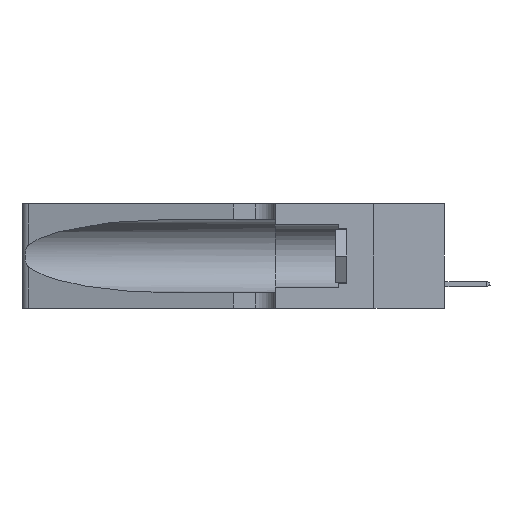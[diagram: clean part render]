
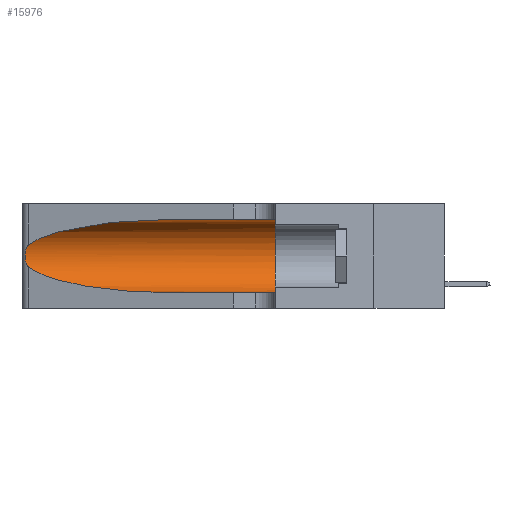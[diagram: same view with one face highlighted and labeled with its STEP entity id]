
A CAD part, left-side view. The second image highlights one B-rep face of the part: STEP entity #15976.
In plain terms, the highlighted cylindrical face has radius 3.308 mm (diameter 6.617 mm), a partial arc.
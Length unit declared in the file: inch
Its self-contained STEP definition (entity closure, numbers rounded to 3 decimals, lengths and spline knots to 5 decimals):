
#788 = CARTESIAN_POINT ( 'NONE',  ( 0.25487, 1.22718, 0.22369 ) ) ;
#1173 = CARTESIAN_POINT ( 'NONE',  ( 0.1305, 0.72297, 0.05475 ) ) ;
#1463 = DIRECTION ( 'NONE',  ( 0., -1., 0. ) ) ;
#1502 = CARTESIAN_POINT ( 'NONE',  ( 0.26018, 1.23835, 0.19895 ) ) ;
#1537 = ORIENTED_EDGE ( 'NONE', *, *, #6121, .T. ) ;
#1835 = VERTEX_POINT ( 'NONE', #3418 ) ;
#2239 = B_SPLINE_CURVE_WITH_KNOTS ( 'NONE', 3,
 ( #13172, #17403, #13436, #3181, #11538, #1502, #15188, #3264, #3517, #17482, #17229, #19241, #7269, #13515 ),
 .UNSPECIFIED., .F., .F.,
 ( 4, 2, 2, 2, 2, 2, 4 ),
 ( 0., 0.00027, 0.00053, 0.00107, 0.0016, 0.00187, 0.00214 ),
 .UNSPECIFIED. ) ;
#2704 = CARTESIAN_POINT ( 'NONE',  ( 0.2373, 1.15595, 0.08982 ) ) ;
#2873 = CARTESIAN_POINT ( 'NONE',  ( 0.25487, 1.22718, 0.14631 ) ) ;
#3123 = VERTEX_POINT ( 'NONE', #2873 ) ;
#3129 = VECTOR ( 'NONE', #4085, 39.37008 ) ;
#3181 = CARTESIAN_POINT ( 'NONE',  ( 0.25787, 1.23484, 0.2124 ) ) ;
#3264 = CARTESIAN_POINT ( 'NONE',  ( 0.26075, 1.23896, 0.178 ) ) ;
#3418 = CARTESIAN_POINT ( 'NONE',  ( 0.1305, 0.35, 0.05475 ) ) ;
#3517 = CARTESIAN_POINT ( 'NONE',  ( 0.26017, 1.23833, 0.17102 ) ) ;
#3657 = CARTESIAN_POINT ( 'NONE',  ( 0.1305, 0.35, 0.185 ) ) ;
#4085 = DIRECTION ( 'NONE',  ( 0., -1., 0. ) ) ;
#4958 = CARTESIAN_POINT ( 'NONE',  ( 0.18966, 0.96281, 0.31525 ) ) ;
#5307 = EDGE_CURVE ( 'NONE', #25484, #12377, #20022, .T. ) ;
#5622 = DIRECTION ( 'NONE',  ( 0., 1., 0. ) ) ;
#6121 = EDGE_CURVE ( 'NONE', #3123, #25502, #10737, .T. ) ;
#6698 = CARTESIAN_POINT ( 'NONE',  ( 0.18966, 0.96281, 0.05475 ) ) ;
#6834 = EDGE_CURVE ( 'NONE', #12377, #3123, #2239, .T. ) ;
#6978 = CARTESIAN_POINT ( 'NONE',  ( 0.2373, 1.15595, 0.28018 ) ) ;
#7135 = VECTOR ( 'NONE', #20220, 39.37008 ) ;
#7269 = CARTESIAN_POINT ( 'NONE',  ( 0.25555, 1.22993, 0.14849 ) ) ;
#7439 = LINE ( 'NONE', #25534, #7135 ) ;
#7719 = DIRECTION ( 'NONE',  ( 0., 0., 1. ) ) ;
#7874 = ORIENTED_EDGE ( 'NONE', *, *, #12235, .F. ) ;
#8394 = LINE ( 'NONE', #21883, #3129 ) ;
#8691 = CARTESIAN_POINT ( 'NONE',  ( 0.1305, 0.72297, 0.05475 ) ) ;
#10331 = EDGE_CURVE ( 'NONE', #25484, #12936, #8394, .T. ) ;
#10737 =( BOUNDED_CURVE ( )  B_SPLINE_CURVE ( 3, ( #25036, #2704, #6698, #8691 ),
 .UNSPECIFIED., .F., .T. ) 
 B_SPLINE_CURVE_WITH_KNOTS ( ( 4, 4 ),
 ( 3.44316, 4.71239 ),
 .UNSPECIFIED. ) 
 CURVE ( )  GEOMETRIC_REPRESENTATION_ITEM ( )  RATIONAL_B_SPLINE_CURVE ( ( 1., 0.87, 0.87, 1. ) ) 
 REPRESENTATION_ITEM ( '' )  );
#11096 = CARTESIAN_POINT ( 'NONE',  ( 0.1305, 0.72297, 0.31525 ) ) ;
#11343 = CARTESIAN_POINT ( 'NONE',  ( 0.25487, 1.22718, 0.22369 ) ) ;
#11538 = CARTESIAN_POINT ( 'NONE',  ( 0.25854, 1.2359, 0.20912 ) ) ;
#11577 = CARTESIAN_POINT ( 'NONE',  ( 0.1305, 1.61858, 0.185 ) ) ;
#11634 = CYLINDRICAL_SURFACE ( 'NONE', #13107, 0.13025 ) ;
#12021 = EDGE_CURVE ( 'NONE', #25502, #1835, #7439, .T. ) ;
#12235 = EDGE_CURVE ( 'NONE', #12936, #1835, #13033, .T. ) ;
#12252 = FACE_OUTER_BOUND ( 'NONE', #20084, .T. ) ;
#12377 = VERTEX_POINT ( 'NONE', #788 ) ;
#12936 = VERTEX_POINT ( 'NONE', #19093 ) ;
#13033 = CIRCLE ( 'NONE', #22105, 0.13025 ) ;
#13107 = AXIS2_PLACEMENT_3D ( 'NONE', #11577, #1463, #23694 ) ;
#13172 = CARTESIAN_POINT ( 'NONE',  ( 0.25487, 1.22718, 0.22369 ) ) ;
#13436 = CARTESIAN_POINT ( 'NONE',  ( 0.25639, 1.23184, 0.21858 ) ) ;
#13515 = CARTESIAN_POINT ( 'NONE',  ( 0.25487, 1.22718, 0.14631 ) ) ;
#13777 = ORIENTED_EDGE ( 'NONE', *, *, #12021, .T. ) ;
#15188 = CARTESIAN_POINT ( 'NONE',  ( 0.26075, 1.23896, 0.19203 ) ) ;
#15976 = ADVANCED_FACE ( 'NONE', ( #12252 ), #11634, .F. ) ;
#17229 = CARTESIAN_POINT ( 'NONE',  ( 0.25789, 1.23486, 0.15765 ) ) ;
#17403 = CARTESIAN_POINT ( 'NONE',  ( 0.25555, 1.22994, 0.2215 ) ) ;
#17482 = CARTESIAN_POINT ( 'NONE',  ( 0.25856, 1.23593, 0.16098 ) ) ;
#17850 = ORIENTED_EDGE ( 'NONE', *, *, #5307, .T. ) ;
#18885 = CARTESIAN_POINT ( 'NONE',  ( 0.1305, 0.72297, 0.31525 ) ) ;
#19093 = CARTESIAN_POINT ( 'NONE',  ( 0.1305, 0.35, 0.31525 ) ) ;
#19241 = CARTESIAN_POINT ( 'NONE',  ( 0.25639, 1.23186, 0.15144 ) ) ;
#20022 =( BOUNDED_CURVE ( )  B_SPLINE_CURVE ( 3, ( #11096, #4958, #6978, #11343 ),
 .UNSPECIFIED., .F., .T. ) 
 B_SPLINE_CURVE_WITH_KNOTS ( ( 4, 4 ),
 ( 1.5708, 2.84003 ),
 .UNSPECIFIED. ) 
 CURVE ( )  GEOMETRIC_REPRESENTATION_ITEM ( )  RATIONAL_B_SPLINE_CURVE ( ( 1., 0.87, 0.87, 1. ) ) 
 REPRESENTATION_ITEM ( '' )  );
#20084 = EDGE_LOOP ( 'NONE', ( #17850, #24731, #1537, #13777, #7874, #23854 ) ) ;
#20220 = DIRECTION ( 'NONE',  ( 0., -1., 0. ) ) ;
#21883 = CARTESIAN_POINT ( 'NONE',  ( 0.1305, 1.61858, 0.31525 ) ) ;
#22105 = AXIS2_PLACEMENT_3D ( 'NONE', #3657, #5622, #7719 ) ;
#23694 = DIRECTION ( 'NONE',  ( 0., 0., -1. ) ) ;
#23854 = ORIENTED_EDGE ( 'NONE', *, *, #10331, .F. ) ;
#24731 = ORIENTED_EDGE ( 'NONE', *, *, #6834, .T. ) ;
#25036 = CARTESIAN_POINT ( 'NONE',  ( 0.25487, 1.22718, 0.14631 ) ) ;
#25484 = VERTEX_POINT ( 'NONE', #18885 ) ;
#25502 = VERTEX_POINT ( 'NONE', #1173 ) ;
#25534 = CARTESIAN_POINT ( 'NONE',  ( 0.1305, 1.61858, 0.05475 ) ) ;
